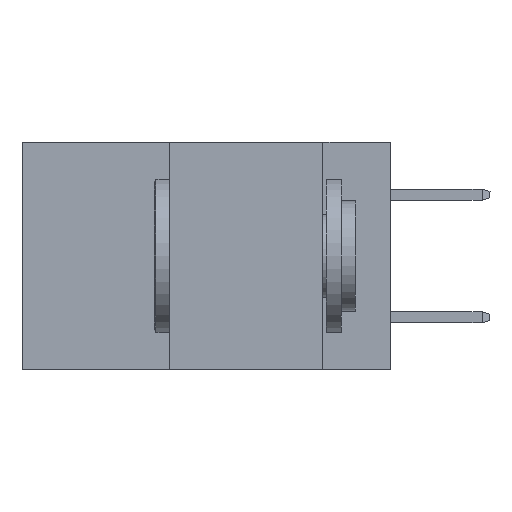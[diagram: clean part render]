
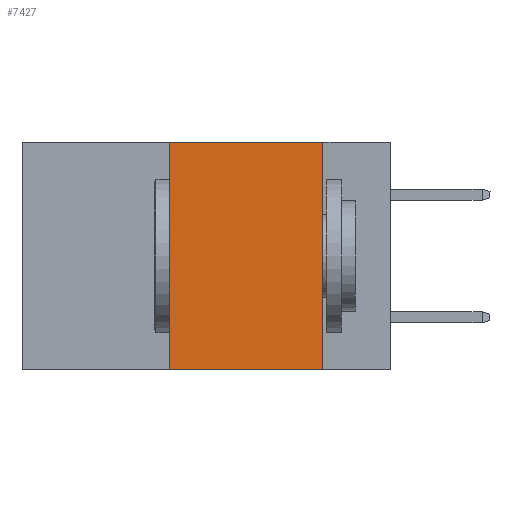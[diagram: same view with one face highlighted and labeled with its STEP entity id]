
A CAD part, left-side view. The second image highlights one B-rep face of the part: STEP entity #7427.
In plain terms, the highlighted planar face has unit normal (-1, 0, 0).
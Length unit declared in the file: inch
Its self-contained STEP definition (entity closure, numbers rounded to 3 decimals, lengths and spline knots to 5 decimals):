
#70 = VERTEX_POINT ( 'NONE', #6538 ) ;
#211 = EDGE_CURVE ( 'NONE', #70, #9503, #2285, .T. ) ;
#276 = LINE ( 'NONE', #2978, #10121 ) ;
#1055 = ORIENTED_EDGE ( 'NONE', *, *, #3461, .F. ) ;
#1865 = CARTESIAN_POINT ( 'NONE',  ( 0., 0.36, -0.37 ) ) ;
#1867 = VECTOR ( 'NONE', #8924, 39.37008 ) ;
#2285 = LINE ( 'NONE', #12173, #1867 ) ;
#2967 = DIRECTION ( 'NONE',  ( 0., -1., 0. ) ) ;
#2978 = CARTESIAN_POINT ( 'NONE',  ( 0., 0.6, 0. ) ) ;
#3257 = LINE ( 'NONE', #11484, #12056 ) ;
#3448 = DIRECTION ( 'NONE',  ( 0., 0., 1. ) ) ;
#3461 = EDGE_CURVE ( 'NONE', #13096, #70, #276, .T. ) ;
#4123 = DIRECTION ( 'NONE',  ( 0., 0., -1. ) ) ;
#4655 = FACE_OUTER_BOUND ( 'NONE', #13149, .T. ) ;
#5652 = CARTESIAN_POINT ( 'NONE',  ( 0., 0.6, -0.37 ) ) ;
#5745 = DIRECTION ( 'NONE',  ( 0., -1., 0. ) ) ;
#6533 = ORIENTED_EDGE ( 'NONE', *, *, #9568, .F. ) ;
#6538 = CARTESIAN_POINT ( 'NONE',  ( 0., 0.11, 0. ) ) ;
#6598 = EDGE_CURVE ( 'NONE', #14866, #9503, #6719, .T. ) ;
#6719 = LINE ( 'NONE', #5652, #9762 ) ;
#6901 = ORIENTED_EDGE ( 'NONE', *, *, #6598, .T. ) ;
#7427 = ADVANCED_FACE ( 'NONE', ( #4655 ), #14217, .F. ) ;
#8031 = CARTESIAN_POINT ( 'NONE',  ( 0., 0.11, -0.37 ) ) ;
#8924 = DIRECTION ( 'NONE',  ( 0., 0., -1. ) ) ;
#9503 = VERTEX_POINT ( 'NONE', #8031 ) ;
#9568 = EDGE_CURVE ( 'NONE', #14866, #13096, #3257, .T. ) ;
#9762 = VECTOR ( 'NONE', #5745, 39.37008 ) ;
#9923 = CARTESIAN_POINT ( 'NONE',  ( 0., 0.6, 0. ) ) ;
#10121 = VECTOR ( 'NONE', #2967, 39.37008 ) ;
#10441 = AXIS2_PLACEMENT_3D ( 'NONE', #9923, #11011, #4123 ) ;
#11011 = DIRECTION ( 'NONE',  ( 1., 0., 0. ) ) ;
#11484 = CARTESIAN_POINT ( 'NONE',  ( 0., 0.36, 0. ) ) ;
#12056 = VECTOR ( 'NONE', #3448, 39.37008 ) ;
#12173 = CARTESIAN_POINT ( 'NONE',  ( 0., 0.11, 0. ) ) ;
#13096 = VERTEX_POINT ( 'NONE', #14503 ) ;
#13149 = EDGE_LOOP ( 'NONE', ( #14826, #1055, #6533, #6901 ) ) ;
#14217 = PLANE ( 'NONE',  #10441 ) ;
#14503 = CARTESIAN_POINT ( 'NONE',  ( 0., 0.36, 0. ) ) ;
#14826 = ORIENTED_EDGE ( 'NONE', *, *, #211, .F. ) ;
#14866 = VERTEX_POINT ( 'NONE', #1865 ) ;
